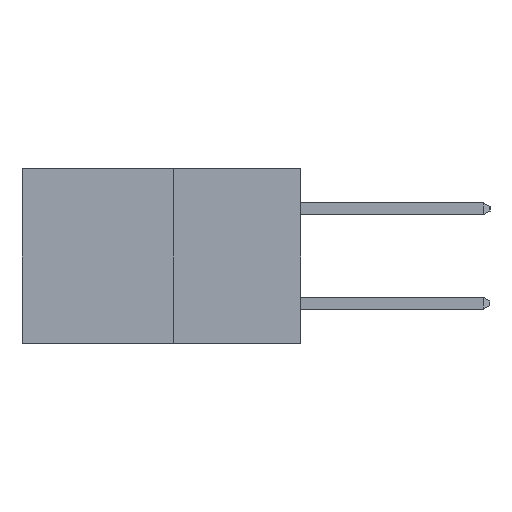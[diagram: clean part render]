
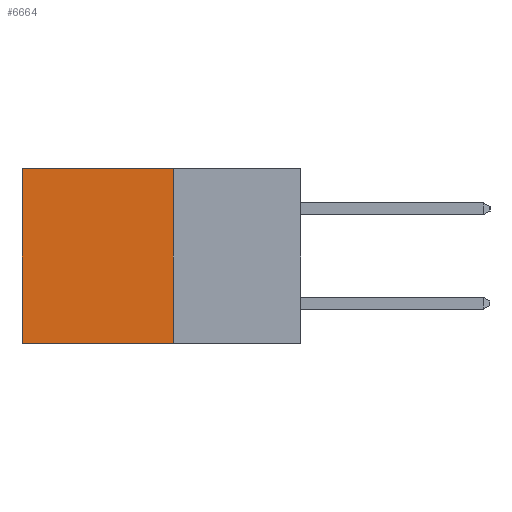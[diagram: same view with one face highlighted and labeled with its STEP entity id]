
A CAD part, left-side view. The second image highlights one B-rep face of the part: STEP entity #6664.
In plain terms, the highlighted planar face has unit normal (-1, 0, 0).
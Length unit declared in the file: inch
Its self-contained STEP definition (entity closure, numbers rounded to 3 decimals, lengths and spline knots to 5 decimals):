
#609 = ORIENTED_EDGE ( 'NONE', *, *, #17599, .F. ) ;
#1304 = AXIS2_PLACEMENT_3D ( 'NONE', #20734, #20710, #20630 ) ;
#1689 = CARTESIAN_POINT ( 'NONE',  ( 0.277, 0.27, -0.37 ) ) ;
#1713 = DIRECTION ( 'NONE',  ( 0., 1., 0. ) ) ;
#2004 = PLANE ( 'NONE',  #1304 ) ;
#4654 = EDGE_CURVE ( 'NONE', #17795, #12685, #10274, .T. ) ;
#4727 = ORIENTED_EDGE ( 'NONE', *, *, #6614, .F. ) ;
#4863 = VECTOR ( 'NONE', #16110, 39.37008 ) ;
#5204 = CARTESIAN_POINT ( 'NONE',  ( 0.277, 0.27, -0.37 ) ) ;
#6126 = CARTESIAN_POINT ( 'NONE',  ( 0.277, 0.27, -0.37 ) ) ;
#6614 = EDGE_CURVE ( 'NONE', #9101, #12685, #15666, .T. ) ;
#6664 = ADVANCED_FACE ( 'NONE', ( #17226 ), #2004, .F. ) ;
#8406 = CARTESIAN_POINT ( 'NONE',  ( 0.277, 0.59, 0. ) ) ;
#8614 = LINE ( 'NONE', #14335, #17958 ) ;
#9101 = VERTEX_POINT ( 'NONE', #5204 ) ;
#9345 = DIRECTION ( 'NONE',  ( 0., 1., 0. ) ) ;
#9362 = LINE ( 'NONE', #6126, #4863 ) ;
#9719 = CARTESIAN_POINT ( 'NONE',  ( 0.277, 0.27, 0. ) ) ;
#10274 = LINE ( 'NONE', #19706, #14155 ) ;
#11392 = EDGE_LOOP ( 'NONE', ( #11557, #4727, #609, #14156 ) ) ;
#11557 = ORIENTED_EDGE ( 'NONE', *, *, #4654, .T. ) ;
#12564 = CARTESIAN_POINT ( 'NONE',  ( 0.277, 0.59, -0.37 ) ) ;
#12685 = VERTEX_POINT ( 'NONE', #12564 ) ;
#12812 = EDGE_CURVE ( 'NONE', #15006, #17795, #8614, .T. ) ;
#14155 = VECTOR ( 'NONE', #19633, 39.37008 ) ;
#14156 = ORIENTED_EDGE ( 'NONE', *, *, #12812, .T. ) ;
#14335 = CARTESIAN_POINT ( 'NONE',  ( 0.277, 0.27, 0. ) ) ;
#15006 = VERTEX_POINT ( 'NONE', #9719 ) ;
#15666 = LINE ( 'NONE', #1689, #20084 ) ;
#16110 = DIRECTION ( 'NONE',  ( 0., 0., -1. ) ) ;
#17226 = FACE_OUTER_BOUND ( 'NONE', #11392, .T. ) ;
#17599 = EDGE_CURVE ( 'NONE', #15006, #9101, #9362, .T. ) ;
#17795 = VERTEX_POINT ( 'NONE', #8406 ) ;
#17958 = VECTOR ( 'NONE', #9345, 39.37008 ) ;
#19633 = DIRECTION ( 'NONE',  ( 0., 0., -1. ) ) ;
#19706 = CARTESIAN_POINT ( 'NONE',  ( 0.277, 0.59, -0.37 ) ) ;
#20084 = VECTOR ( 'NONE', #1713, 39.37008 ) ;
#20630 = DIRECTION ( 'NONE',  ( 0., 0., -1. ) ) ;
#20710 = DIRECTION ( 'NONE',  ( 1., 0., 0. ) ) ;
#20734 = CARTESIAN_POINT ( 'NONE',  ( 0.277, 0.27, -0.37 ) ) ;
